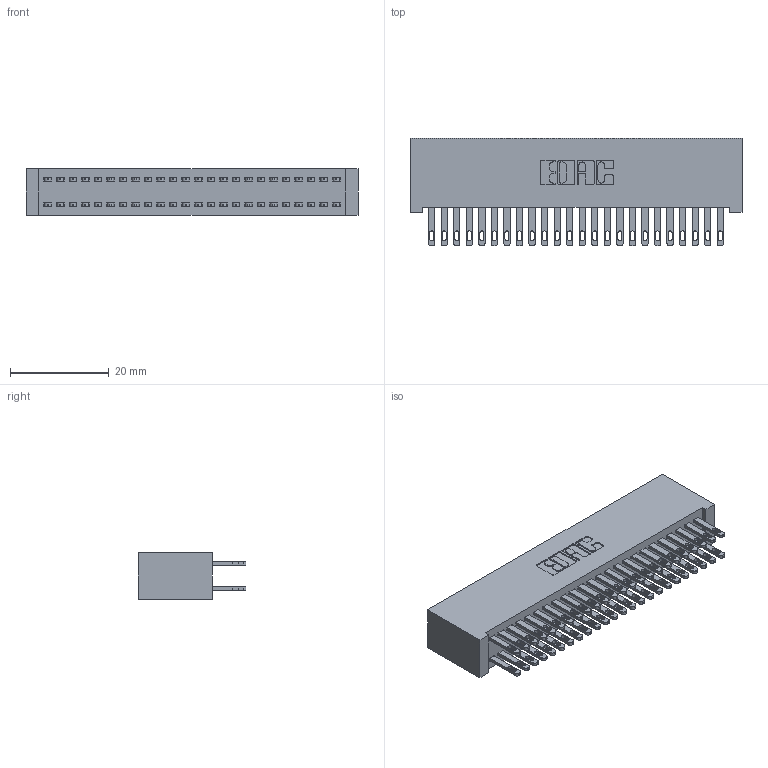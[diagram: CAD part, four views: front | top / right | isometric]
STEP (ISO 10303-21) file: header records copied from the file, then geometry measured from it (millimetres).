
FILE_DESCRIPTION (( 'STEP AP203' ), '1' );
FILE_NAME ('892-048-500-201.STEP', '2020-09-21T17:32:59', ( '' ), ( '' ), 'SwSTEP 2.0', 'SolidWorks 2020', '' );
FILE_SCHEMA (( 'CONFIG_CONTROL_DESIGN' ));
Length unit declared in the file: inch
Products named in the file (3): 345-292-001_345-293-100; 842 Part_Lugless; 892-048-500-201
Assembly tree (49 placements, depth 2):
  892-048-500-201
    842 Part_Lugless
    345-292-001_345-293-100  x48
Bounding box: 67.21 x 21.85 x 9.4 mm (x, y, z)
Volume: 6539.7 mm3; surface area: 11107.2 mm2
Topology: 49 solids, 49 shells, 2406 faces, 7331 edges, 4886 vertices
Faces by surface type: plane 1502, cylinder 904
Entity records: 17289 total; most frequent: CARTESIAN_POINT 2882, ORIENTED_EDGE 2818, DIRECTION 2489, EDGE_CURVE 1409, VECTOR 1285, LINE 1285, VERTEX_POINT 938, AXIS2_PLACEMENT_3D 602
